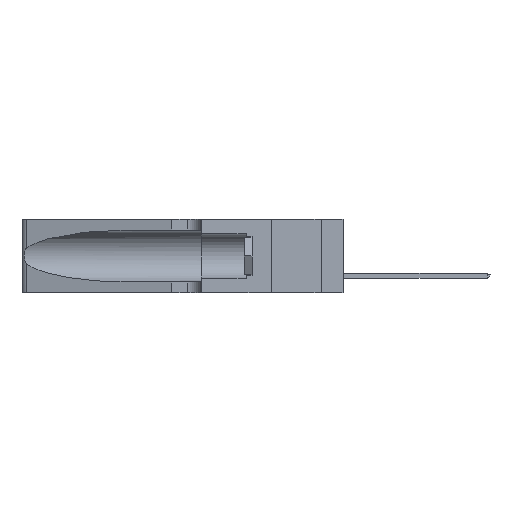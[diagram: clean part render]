
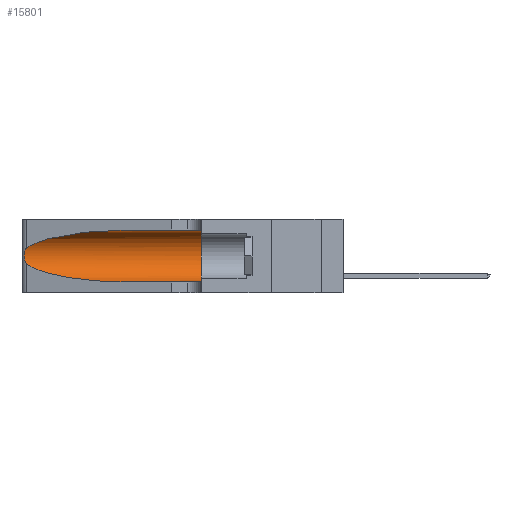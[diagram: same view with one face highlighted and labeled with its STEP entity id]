
A CAD part, left-side view. The second image highlights one B-rep face of the part: STEP entity #15801.
In plain terms, the highlighted cylindrical face has radius 3.308 mm (diameter 6.617 mm), a partial arc.
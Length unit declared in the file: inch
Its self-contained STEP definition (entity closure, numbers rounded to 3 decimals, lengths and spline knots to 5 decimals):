
#2057 = ORIENTED_EDGE ( 'NONE', *, *, #50291, .F. ) ;
#2529 = CARTESIAN_POINT ( 'NONE',  ( 0.25639, 1.23184, 0.21858 ) ) ;
#2533 = DIRECTION ( 'NONE',  ( 0., 0., -1. ) ) ;
#2669 = EDGE_CURVE ( 'NONE', #35954, #45062, #19985, .T. ) ;
#2706 = CARTESIAN_POINT ( 'NONE',  ( 0.1305, 1.61858, 0.185 ) ) ;
#3058 = CARTESIAN_POINT ( 'NONE',  ( 0.25487, 1.22718, 0.22369 ) ) ;
#3213 = FACE_OUTER_BOUND ( 'NONE', #25046, .T. ) ;
#3393 = CARTESIAN_POINT ( 'NONE',  ( 0.26075, 1.23896, 0.178 ) ) ;
#4200 = CARTESIAN_POINT ( 'NONE',  ( 0.1305, 1.61858, 0.05475 ) ) ;
#5894 = DIRECTION ( 'NONE',  ( 0., -1., 0. ) ) ;
#8022 = AXIS2_PLACEMENT_3D ( 'NONE', #9946, #17630, #21943 ) ;
#8791 = EDGE_CURVE ( 'NONE', #35954, #13000, #47884, .T. ) ;
#9434 = CARTESIAN_POINT ( 'NONE',  ( 0.25487, 1.22718, 0.14631 ) ) ;
#9946 = CARTESIAN_POINT ( 'NONE',  ( 0.1305, 0.35, 0.185 ) ) ;
#10481 = CARTESIAN_POINT ( 'NONE',  ( 0.25487, 1.22718, 0.22369 ) ) ;
#10759 = ORIENTED_EDGE ( 'NONE', *, *, #17196, .T. ) ;
#12451 = ORIENTED_EDGE ( 'NONE', *, *, #39142, .T. ) ;
#13000 = VERTEX_POINT ( 'NONE', #10481 ) ;
#13735 = CARTESIAN_POINT ( 'NONE',  ( 0.2373, 1.15595, 0.28018 ) ) ;
#13908 = CARTESIAN_POINT ( 'NONE',  ( 0.1305, 0.72297, 0.31525 ) ) ;
#14473 = CARTESIAN_POINT ( 'NONE',  ( 0.1305, 0.35, 0.31525 ) ) ;
#15801 = ADVANCED_FACE ( 'NONE', ( #3213 ), #31842, .F. ) ;
#16676 = LINE ( 'NONE', #4200, #37522 ) ;
#17196 = EDGE_CURVE ( 'NONE', #13000, #29183, #28870, .T. ) ;
#17341 = CARTESIAN_POINT ( 'NONE',  ( 0.18966, 0.96281, 0.05475 ) ) ;
#17630 = DIRECTION ( 'NONE',  ( 0., 1., 0. ) ) ;
#18704 = CARTESIAN_POINT ( 'NONE',  ( 0.1305, 0.72297, 0.05475 ) ) ;
#19985 = LINE ( 'NONE', #49514, #39537 ) ;
#20539 = CARTESIAN_POINT ( 'NONE',  ( 0.1305, 0.72297, 0.31525 ) ) ;
#20700 =( BOUNDED_CURVE ( )  B_SPLINE_CURVE ( 3, ( #48030, #24839, #17341, #36979 ),
 .UNSPECIFIED., .F., .T. ) 
 B_SPLINE_CURVE_WITH_KNOTS ( ( 4, 4 ),
 ( 3.44316, 4.71239 ),
 .UNSPECIFIED. ) 
 CURVE ( )  GEOMETRIC_REPRESENTATION_ITEM ( )  RATIONAL_B_SPLINE_CURVE ( ( 1., 0.87, 0.87, 1. ) ) 
 REPRESENTATION_ITEM ( '' )  );
#21943 = DIRECTION ( 'NONE',  ( 0., 0., 1. ) ) ;
#24598 = ORIENTED_EDGE ( 'NONE', *, *, #8791, .T. ) ;
#24839 = CARTESIAN_POINT ( 'NONE',  ( 0.2373, 1.15595, 0.08982 ) ) ;
#25046 = EDGE_LOOP ( 'NONE', ( #24598, #10759, #12451, #41452, #2057, #25124 ) ) ;
#25095 = VERTEX_POINT ( 'NONE', #37737 ) ;
#25124 = ORIENTED_EDGE ( 'NONE', *, *, #2669, .F. ) ;
#28870 = B_SPLINE_CURVE_WITH_KNOTS ( 'NONE', 3,
 ( #3058, #30411, #2529, #29879, #49505, #34329, #30062, #3393, #44986, #39391, #43603, #48185, #35928, #9434 ),
 .UNSPECIFIED., .F., .F.,
 ( 4, 2, 2, 2, 2, 2, 4 ),
 ( 0., 0.00027, 0.00053, 0.00107, 0.0016, 0.00187, 0.00214 ),
 .UNSPECIFIED. ) ;
#29183 = VERTEX_POINT ( 'NONE', #48504 ) ;
#29879 = CARTESIAN_POINT ( 'NONE',  ( 0.25787, 1.23484, 0.2124 ) ) ;
#30062 = CARTESIAN_POINT ( 'NONE',  ( 0.26075, 1.23896, 0.19203 ) ) ;
#30411 = CARTESIAN_POINT ( 'NONE',  ( 0.25555, 1.22994, 0.2215 ) ) ;
#30883 = VERTEX_POINT ( 'NONE', #18704 ) ;
#31842 = CYLINDRICAL_SURFACE ( 'NONE', #37850, 0.13025 ) ;
#33462 = DIRECTION ( 'NONE',  ( 0., -1., 0. ) ) ;
#34329 = CARTESIAN_POINT ( 'NONE',  ( 0.26018, 1.23835, 0.19895 ) ) ;
#35578 = DIRECTION ( 'NONE',  ( 0., -1., 0. ) ) ;
#35928 = CARTESIAN_POINT ( 'NONE',  ( 0.25555, 1.22993, 0.14849 ) ) ;
#35954 = VERTEX_POINT ( 'NONE', #13908 ) ;
#36979 = CARTESIAN_POINT ( 'NONE',  ( 0.1305, 0.72297, 0.05475 ) ) ;
#37522 = VECTOR ( 'NONE', #35578, 39.37008 ) ;
#37737 = CARTESIAN_POINT ( 'NONE',  ( 0.1305, 0.35, 0.05475 ) ) ;
#37850 = AXIS2_PLACEMENT_3D ( 'NONE', #2706, #5894, #2533 ) ;
#39142 = EDGE_CURVE ( 'NONE', #29183, #30883, #20700, .T. ) ;
#39391 = CARTESIAN_POINT ( 'NONE',  ( 0.25856, 1.23593, 0.16098 ) ) ;
#39537 = VECTOR ( 'NONE', #33462, 39.37008 ) ;
#41452 = ORIENTED_EDGE ( 'NONE', *, *, #46715, .T. ) ;
#43603 = CARTESIAN_POINT ( 'NONE',  ( 0.25789, 1.23486, 0.15765 ) ) ;
#44986 = CARTESIAN_POINT ( 'NONE',  ( 0.26017, 1.23833, 0.17102 ) ) ;
#45062 = VERTEX_POINT ( 'NONE', #14473 ) ;
#45701 = CARTESIAN_POINT ( 'NONE',  ( 0.18966, 0.96281, 0.31525 ) ) ;
#46715 = EDGE_CURVE ( 'NONE', #30883, #25095, #16676, .T. ) ;
#47884 =( BOUNDED_CURVE ( )  B_SPLINE_CURVE ( 3, ( #20539, #45701, #13735, #49952 ),
 .UNSPECIFIED., .F., .F. ) 
 B_SPLINE_CURVE_WITH_KNOTS ( ( 4, 4 ),
 ( 1.5708, 2.84003 ),
 .UNSPECIFIED. ) 
 CURVE ( )  GEOMETRIC_REPRESENTATION_ITEM ( )  RATIONAL_B_SPLINE_CURVE ( ( 1., 0.87, 0.87, 1. ) ) 
 REPRESENTATION_ITEM ( '' )  );
#48030 = CARTESIAN_POINT ( 'NONE',  ( 0.25487, 1.22718, 0.14631 ) ) ;
#48185 = CARTESIAN_POINT ( 'NONE',  ( 0.25639, 1.23186, 0.15144 ) ) ;
#48504 = CARTESIAN_POINT ( 'NONE',  ( 0.25487, 1.22718, 0.14631 ) ) ;
#49153 = CIRCLE ( 'NONE', #8022, 0.13025 ) ;
#49505 = CARTESIAN_POINT ( 'NONE',  ( 0.25854, 1.2359, 0.20912 ) ) ;
#49514 = CARTESIAN_POINT ( 'NONE',  ( 0.1305, 1.61858, 0.31525 ) ) ;
#49952 = CARTESIAN_POINT ( 'NONE',  ( 0.25487, 1.22718, 0.22369 ) ) ;
#50291 = EDGE_CURVE ( 'NONE', #45062, #25095, #49153, .T. ) ;
